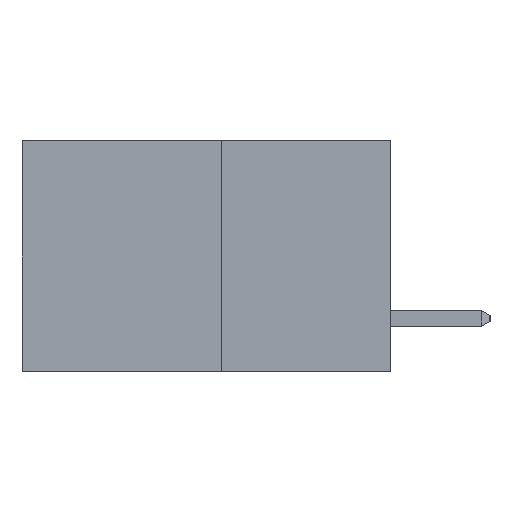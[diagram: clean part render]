
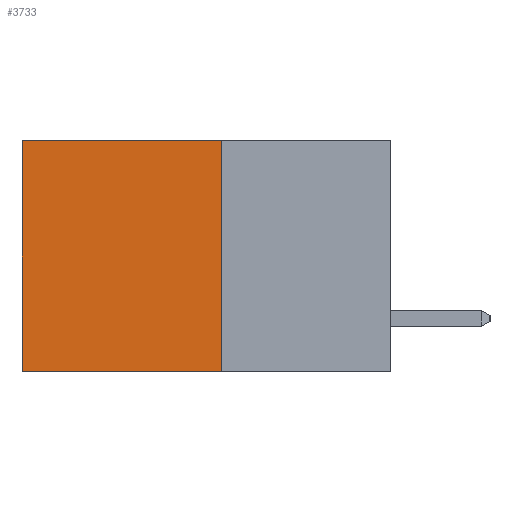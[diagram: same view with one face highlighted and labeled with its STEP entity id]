
A CAD part, left-side view. The second image highlights one B-rep face of the part: STEP entity #3733.
In plain terms, the highlighted planar face has unit normal (-1, 0, 0).
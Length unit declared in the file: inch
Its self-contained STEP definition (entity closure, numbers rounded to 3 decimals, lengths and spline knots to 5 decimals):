
#237 = EDGE_CURVE ( 'NONE', #1962, #5282, #8544, .T. ) ;
#448 = DIRECTION ( 'NONE',  ( 0., 0., -1. ) ) ;
#646 = VECTOR ( 'NONE', #5266, 39.37008 ) ;
#875 = PLANE ( 'NONE',  #10043 ) ;
#1178 = LINE ( 'NONE', #1646, #646 ) ;
#1327 = CARTESIAN_POINT ( 'NONE',  ( 0.277, 0.27, 0. ) ) ;
#1646 = CARTESIAN_POINT ( 'NONE',  ( 0.277, 0.27, -0.37 ) ) ;
#1707 = DIRECTION ( 'NONE',  ( 1., 0., 0. ) ) ;
#1882 = VECTOR ( 'NONE', #6148, 39.37008 ) ;
#1962 = VERTEX_POINT ( 'NONE', #5205 ) ;
#2490 = VECTOR ( 'NONE', #7052, 39.37008 ) ;
#2766 = LINE ( 'NONE', #6264, #2490 ) ;
#2924 = EDGE_CURVE ( 'NONE', #6904, #5282, #1178, .T. ) ;
#3733 = ADVANCED_FACE ( 'NONE', ( #3741 ), #875, .F. ) ;
#3741 = FACE_OUTER_BOUND ( 'NONE', #9583, .T. ) ;
#4028 = ORIENTED_EDGE ( 'NONE', *, *, #6785, .T. ) ;
#4261 = ORIENTED_EDGE ( 'NONE', *, *, #10282, .F. ) ;
#4596 = CARTESIAN_POINT ( 'NONE',  ( 0.277, 0.27, -0.37 ) ) ;
#4743 = ORIENTED_EDGE ( 'NONE', *, *, #2924, .F. ) ;
#4750 = CARTESIAN_POINT ( 'NONE',  ( 0.277, 0.27, -0.37 ) ) ;
#4991 = ORIENTED_EDGE ( 'NONE', *, *, #237, .T. ) ;
#5205 = CARTESIAN_POINT ( 'NONE',  ( 0.277, 0.59, 0. ) ) ;
#5266 = DIRECTION ( 'NONE',  ( 0., 1., 0. ) ) ;
#5282 = VERTEX_POINT ( 'NONE', #9978 ) ;
#5805 = CARTESIAN_POINT ( 'NONE',  ( 0.277, 0.27, -0.37 ) ) ;
#6148 = DIRECTION ( 'NONE',  ( 0., 0., -1. ) ) ;
#6264 = CARTESIAN_POINT ( 'NONE',  ( 0.277, 0.27, 0. ) ) ;
#6785 = EDGE_CURVE ( 'NONE', #7389, #1962, #2766, .T. ) ;
#6904 = VERTEX_POINT ( 'NONE', #4750 ) ;
#7052 = DIRECTION ( 'NONE',  ( 0., 1., 0. ) ) ;
#7389 = VERTEX_POINT ( 'NONE', #1327 ) ;
#7395 = DIRECTION ( 'NONE',  ( 0., 0., -1. ) ) ;
#8284 = LINE ( 'NONE', #4596, #9756 ) ;
#8544 = LINE ( 'NONE', #8655, #1882 ) ;
#8655 = CARTESIAN_POINT ( 'NONE',  ( 0.277, 0.59, -0.37 ) ) ;
#9583 = EDGE_LOOP ( 'NONE', ( #4991, #4743, #4261, #4028 ) ) ;
#9756 = VECTOR ( 'NONE', #448, 39.37008 ) ;
#9978 = CARTESIAN_POINT ( 'NONE',  ( 0.277, 0.59, -0.37 ) ) ;
#10043 = AXIS2_PLACEMENT_3D ( 'NONE', #5805, #1707, #7395 ) ;
#10282 = EDGE_CURVE ( 'NONE', #7389, #6904, #8284, .T. ) ;
